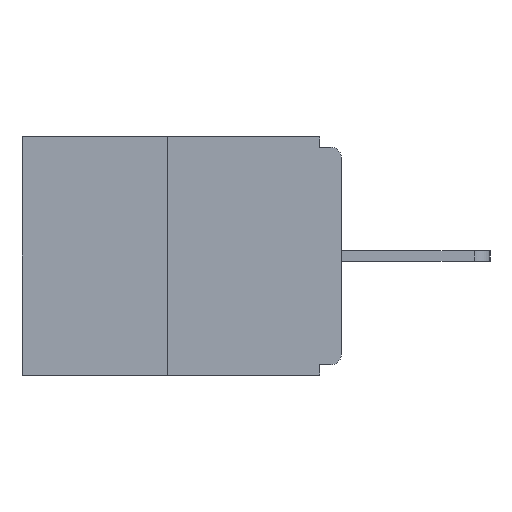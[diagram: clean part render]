
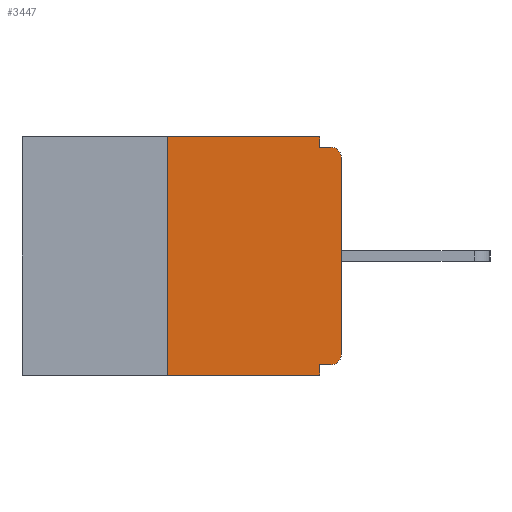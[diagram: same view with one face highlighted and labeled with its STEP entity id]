
A CAD part, left-side view. The second image highlights one B-rep face of the part: STEP entity #3447.
In plain terms, the highlighted planar face has unit normal (-1, 0, 0).
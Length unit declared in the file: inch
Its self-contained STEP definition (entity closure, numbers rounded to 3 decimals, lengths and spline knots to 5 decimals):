
#112 = LINE ( 'NONE', #1715, #14513 ) ;
#528 = LINE ( 'NONE', #5395, #16177 ) ;
#565 = ORIENTED_EDGE ( 'NONE', *, *, #8353, .T. ) ;
#728 = DIRECTION ( 'NONE',  ( 0., 0., -1. ) ) ;
#841 = CARTESIAN_POINT ( 'NONE',  ( 0., 0.015, -0.328 ) ) ;
#1307 = CARTESIAN_POINT ( 'NONE',  ( 0., 0.46, -0.343 ) ) ;
#1399 = CARTESIAN_POINT ( 'NONE',  ( 0., 0., -0.015 ) ) ;
#1423 = ORIENTED_EDGE ( 'NONE', *, *, #3425, .T. ) ;
#1449 = DIRECTION ( 'NONE',  ( 0., -1., 0. ) ) ;
#1687 = LINE ( 'NONE', #1399, #16758 ) ;
#1715 = CARTESIAN_POINT ( 'NONE',  ( 0., 0.25, 0. ) ) ;
#1820 = VERTEX_POINT ( 'NONE', #6655 ) ;
#1896 = ORIENTED_EDGE ( 'NONE', *, *, #11086, .F. ) ;
#1926 = EDGE_CURVE ( 'NONE', #4287, #8063, #1687, .T. ) ;
#2680 = CARTESIAN_POINT ( 'NONE',  ( 0., 0.25, 0. ) ) ;
#3425 = EDGE_CURVE ( 'NONE', #15394, #3869, #12865, .T. ) ;
#3447 = ADVANCED_FACE ( 'NONE', ( #8169 ), #5086, .F. ) ;
#3457 = CARTESIAN_POINT ( 'NONE',  ( 0., 0.031, -0.015 ) ) ;
#3545 = CARTESIAN_POINT ( 'NONE',  ( 0., 0.46, 0. ) ) ;
#3629 = DIRECTION ( 'NONE',  ( 0., 0., -1. ) ) ;
#3869 = VERTEX_POINT ( 'NONE', #6086 ) ;
#4123 = VERTEX_POINT ( 'NONE', #2680 ) ;
#4267 = VECTOR ( 'NONE', #728, 39.37008 ) ;
#4287 = VERTEX_POINT ( 'NONE', #3457 ) ;
#4407 = CARTESIAN_POINT ( 'NONE',  ( 0., 0.031, 0. ) ) ;
#4413 = EDGE_CURVE ( 'NONE', #1820, #5958, #16941, .T. ) ;
#4649 = DIRECTION ( 'NONE',  ( -1., 0., 0. ) ) ;
#4945 = DIRECTION ( 'NONE',  ( -1., 0., 0. ) ) ;
#5086 = PLANE ( 'NONE',  #6012 ) ;
#5306 = VECTOR ( 'NONE', #10762, 39.37008 ) ;
#5395 = CARTESIAN_POINT ( 'NONE',  ( 0., 0., -0.328 ) ) ;
#5958 = VERTEX_POINT ( 'NONE', #7150 ) ;
#6012 = AXIS2_PLACEMENT_3D ( 'NONE', #10535, #7833, #12913 ) ;
#6051 = VECTOR ( 'NONE', #17059, 39.37008 ) ;
#6086 = CARTESIAN_POINT ( 'NONE',  ( 0., 0., -0.03 ) ) ;
#6225 = DIRECTION ( 'NONE',  ( 0., 0., -1. ) ) ;
#6426 = ORIENTED_EDGE ( 'NONE', *, *, #13667, .T. ) ;
#6607 = LINE ( 'NONE', #7294, #4267 ) ;
#6655 = CARTESIAN_POINT ( 'NONE',  ( 0., 0.031, -0.328 ) ) ;
#7150 = CARTESIAN_POINT ( 'NONE',  ( 0., 0.031, -0.343 ) ) ;
#7294 = CARTESIAN_POINT ( 'NONE',  ( 0., 0.031, 0. ) ) ;
#7334 = EDGE_CURVE ( 'NONE', #8464, #1820, #528, .T. ) ;
#7641 = EDGE_LOOP ( 'NONE', ( #9583, #14622, #11512, #14647, #13150, #565, #1423, #6426, #12533, #1896 ) ) ;
#7833 = DIRECTION ( 'NONE',  ( 1., 0., 0. ) ) ;
#8063 = VERTEX_POINT ( 'NONE', #11627 ) ;
#8169 = FACE_OUTER_BOUND ( 'NONE', #7641, .T. ) ;
#8209 = DIRECTION ( 'NONE',  ( 0., 0., 1. ) ) ;
#8353 = EDGE_CURVE ( 'NONE', #8464, #15394, #13519, .T. ) ;
#8464 = VERTEX_POINT ( 'NONE', #841 ) ;
#9007 = CIRCLE ( 'NONE', #9466, 0.015 ) ;
#9466 = AXIS2_PLACEMENT_3D ( 'NONE', #12826, #4945, #6225 ) ;
#9583 = ORIENTED_EDGE ( 'NONE', *, *, #13687, .F. ) ;
#9631 = AXIS2_PLACEMENT_3D ( 'NONE', #9994, #4649, #13924 ) ;
#9994 = CARTESIAN_POINT ( 'NONE',  ( 0., 0.015, -0.313 ) ) ;
#10303 = CARTESIAN_POINT ( 'NONE',  ( 0., 0.031, -0.343 ) ) ;
#10535 = CARTESIAN_POINT ( 'NONE',  ( 0., 0.46, 0. ) ) ;
#10540 = CARTESIAN_POINT ( 'NONE',  ( 0., 0.25, -0.343 ) ) ;
#10762 = DIRECTION ( 'NONE',  ( 0., -1., 0. ) ) ;
#11086 = EDGE_CURVE ( 'NONE', #12583, #4287, #6607, .T. ) ;
#11462 = DIRECTION ( 'NONE',  ( 0., -1., 0. ) ) ;
#11512 = ORIENTED_EDGE ( 'NONE', *, *, #15143, .T. ) ;
#11627 = CARTESIAN_POINT ( 'NONE',  ( 0., 0.015, -0.015 ) ) ;
#12384 = VERTEX_POINT ( 'NONE', #10540 ) ;
#12533 = ORIENTED_EDGE ( 'NONE', *, *, #1926, .F. ) ;
#12583 = VERTEX_POINT ( 'NONE', #4407 ) ;
#12631 = CARTESIAN_POINT ( 'NONE',  ( 0., 0., -0.313 ) ) ;
#12826 = CARTESIAN_POINT ( 'NONE',  ( 0., 0.015, -0.03 ) ) ;
#12865 = LINE ( 'NONE', #12982, #6051 ) ;
#12913 = DIRECTION ( 'NONE',  ( 0., 0., -1. ) ) ;
#12982 = CARTESIAN_POINT ( 'NONE',  ( 0., 0., 0. ) ) ;
#13150 = ORIENTED_EDGE ( 'NONE', *, *, #7334, .F. ) ;
#13307 = EDGE_CURVE ( 'NONE', #12384, #4123, #112, .T. ) ;
#13519 = CIRCLE ( 'NONE', #9631, 0.015 ) ;
#13667 = EDGE_CURVE ( 'NONE', #3869, #8063, #9007, .T. ) ;
#13687 = EDGE_CURVE ( 'NONE', #4123, #12583, #16537, .T. ) ;
#13924 = DIRECTION ( 'NONE',  ( 0., 0., -1. ) ) ;
#14513 = VECTOR ( 'NONE', #8209, 39.37008 ) ;
#14622 = ORIENTED_EDGE ( 'NONE', *, *, #13307, .F. ) ;
#14647 = ORIENTED_EDGE ( 'NONE', *, *, #4413, .F. ) ;
#14869 = VECTOR ( 'NONE', #3629, 39.37008 ) ;
#15143 = EDGE_CURVE ( 'NONE', #12384, #5958, #15344, .T. ) ;
#15344 = LINE ( 'NONE', #1307, #5306 ) ;
#15394 = VERTEX_POINT ( 'NONE', #12631 ) ;
#15957 = DIRECTION ( 'NONE',  ( 0., 1., 0. ) ) ;
#16129 = VECTOR ( 'NONE', #11462, 39.37008 ) ;
#16177 = VECTOR ( 'NONE', #15957, 39.37008 ) ;
#16537 = LINE ( 'NONE', #3545, #16129 ) ;
#16758 = VECTOR ( 'NONE', #1449, 39.37008 ) ;
#16941 = LINE ( 'NONE', #10303, #14869 ) ;
#17059 = DIRECTION ( 'NONE',  ( 0., 0., 1. ) ) ;
